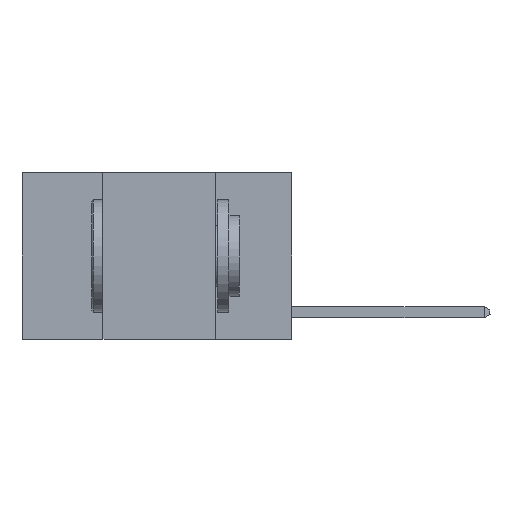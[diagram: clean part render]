
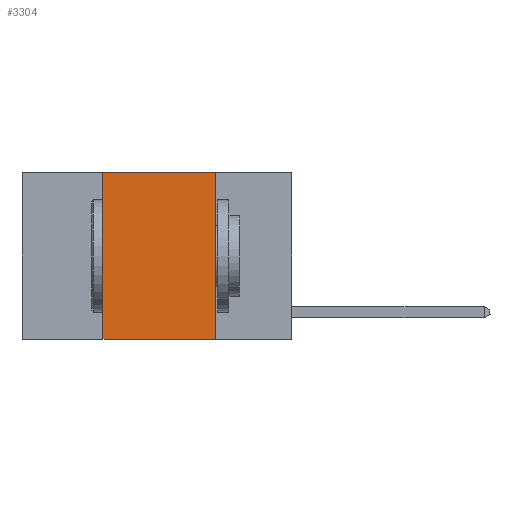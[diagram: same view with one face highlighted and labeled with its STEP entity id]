
A CAD part, left-side view. The second image highlights one B-rep face of the part: STEP entity #3304.
In plain terms, the highlighted planar face has unit normal (-1, 0, 0).
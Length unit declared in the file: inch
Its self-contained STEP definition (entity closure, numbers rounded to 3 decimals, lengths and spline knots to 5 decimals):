
#37 = PLANE ( 'NONE',  #9092 ) ;
#262 = LINE ( 'NONE', #3849, #2197 ) ;
#1507 = CARTESIAN_POINT ( 'NONE',  ( 0., 0.6, -0.37 ) ) ;
#1521 = VECTOR ( 'NONE', #2996, 39.37008 ) ;
#1726 = VECTOR ( 'NONE', #11024, 39.37008 ) ;
#1792 = DIRECTION ( 'NONE',  ( 0., 0., -1. ) ) ;
#2122 = VERTEX_POINT ( 'NONE', #6873 ) ;
#2197 = VECTOR ( 'NONE', #5687, 39.37008 ) ;
#2805 = LINE ( 'NONE', #5221, #5061 ) ;
#2996 = DIRECTION ( 'NONE',  ( 0., 0., 1. ) ) ;
#3108 = VERTEX_POINT ( 'NONE', #8197 ) ;
#3304 = ADVANCED_FACE ( 'NONE', ( #10187 ), #37, .F. ) ;
#3849 = CARTESIAN_POINT ( 'NONE',  ( 0., 0.6, 0. ) ) ;
#4273 = EDGE_CURVE ( 'NONE', #3108, #4630, #262, .T. ) ;
#4630 = VERTEX_POINT ( 'NONE', #11786 ) ;
#5061 = VECTOR ( 'NONE', #6556, 39.37008 ) ;
#5221 = CARTESIAN_POINT ( 'NONE',  ( 0., 0.17, 0. ) ) ;
#5418 = CARTESIAN_POINT ( 'NONE',  ( 0., 0.6, 0. ) ) ;
#5630 = CARTESIAN_POINT ( 'NONE',  ( 0., 0.42, 0. ) ) ;
#5687 = DIRECTION ( 'NONE',  ( 0., -1., 0. ) ) ;
#6556 = DIRECTION ( 'NONE',  ( 0., 0., -1. ) ) ;
#6873 = CARTESIAN_POINT ( 'NONE',  ( 0., 0.17, -0.37 ) ) ;
#8158 = EDGE_LOOP ( 'NONE', ( #10588, #9289, #10209, #11928 ) ) ;
#8197 = CARTESIAN_POINT ( 'NONE',  ( 0., 0.42, 0. ) ) ;
#8260 = DIRECTION ( 'NONE',  ( 1., 0., 0. ) ) ;
#9092 = AXIS2_PLACEMENT_3D ( 'NONE', #5418, #8260, #1792 ) ;
#9289 = ORIENTED_EDGE ( 'NONE', *, *, #4273, .F. ) ;
#10187 = FACE_OUTER_BOUND ( 'NONE', #8158, .T. ) ;
#10209 = ORIENTED_EDGE ( 'NONE', *, *, #10340, .F. ) ;
#10340 = EDGE_CURVE ( 'NONE', #10998, #3108, #11467, .T. ) ;
#10588 = ORIENTED_EDGE ( 'NONE', *, *, #11317, .F. ) ;
#10863 = EDGE_CURVE ( 'NONE', #10998, #2122, #10957, .T. ) ;
#10957 = LINE ( 'NONE', #1507, #1726 ) ;
#10998 = VERTEX_POINT ( 'NONE', #12106 ) ;
#11024 = DIRECTION ( 'NONE',  ( 0., -1., 0. ) ) ;
#11317 = EDGE_CURVE ( 'NONE', #4630, #2122, #2805, .T. ) ;
#11467 = LINE ( 'NONE', #5630, #1521 ) ;
#11786 = CARTESIAN_POINT ( 'NONE',  ( 0., 0.17, 0. ) ) ;
#11928 = ORIENTED_EDGE ( 'NONE', *, *, #10863, .T. ) ;
#12106 = CARTESIAN_POINT ( 'NONE',  ( 0., 0.42, -0.37 ) ) ;
